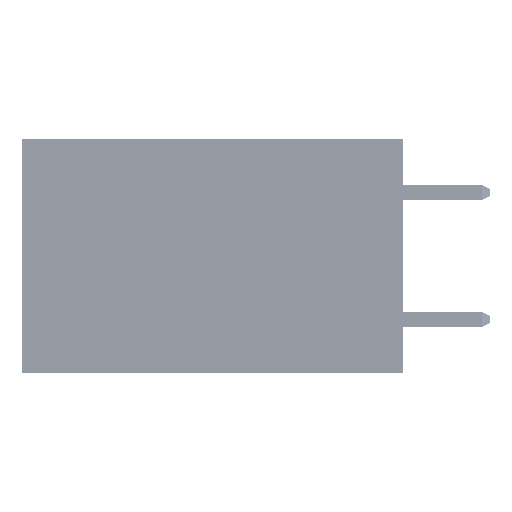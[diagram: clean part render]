
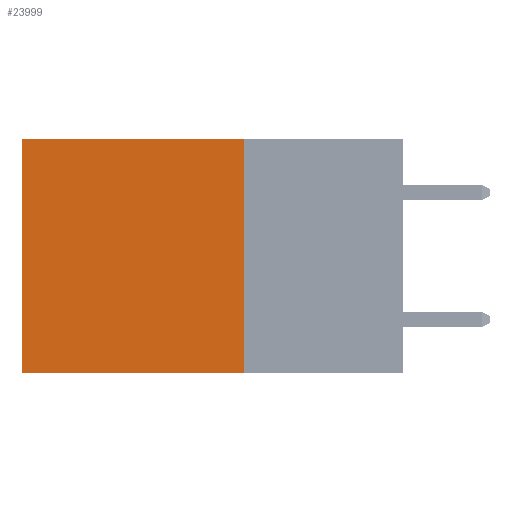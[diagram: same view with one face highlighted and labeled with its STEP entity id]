
A CAD part, left-side view. The second image highlights one B-rep face of the part: STEP entity #23999.
In plain terms, the highlighted planar face has unit normal (-1, 0, 0).
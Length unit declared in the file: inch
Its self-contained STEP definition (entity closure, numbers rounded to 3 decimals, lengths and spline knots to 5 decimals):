
#583 = EDGE_CURVE ( 'NONE', #38923, #5030, #13381, .T. ) ;
#1018 = DIRECTION ( 'NONE',  ( 0., 0., -1. ) ) ;
#1127 = DIRECTION ( 'NONE',  ( 0., 1., 0. ) ) ;
#1425 = CARTESIAN_POINT ( 'NONE',  ( 0.2875, 0.6, -0.37 ) ) ;
#4219 = ORIENTED_EDGE ( 'NONE', *, *, #45315, .T. ) ;
#4636 = ORIENTED_EDGE ( 'NONE', *, *, #12246, .T. ) ;
#5030 = VERTEX_POINT ( 'NONE', #37125 ) ;
#11521 = CARTESIAN_POINT ( 'NONE',  ( 0.2875, 0.6, 0. ) ) ;
#12246 = EDGE_CURVE ( 'NONE', #23086, #42691, #13013, .T. ) ;
#13013 = LINE ( 'NONE', #37591, #28903 ) ;
#13381 = LINE ( 'NONE', #17433, #22568 ) ;
#14791 = VECTOR ( 'NONE', #41757, 39.37008 ) ;
#17433 = CARTESIAN_POINT ( 'NONE',  ( 0.2875, 0.25, 0. ) ) ;
#17654 = DIRECTION ( 'NONE',  ( 0., 0., -1. ) ) ;
#18188 = ORIENTED_EDGE ( 'NONE', *, *, #583, .F. ) ;
#19488 = VECTOR ( 'NONE', #1127, 39.37008 ) ;
#19728 = FACE_OUTER_BOUND ( 'NONE', #33648, .T. ) ;
#22568 = VECTOR ( 'NONE', #35327, 39.37008 ) ;
#23086 = VERTEX_POINT ( 'NONE', #11521 ) ;
#23753 = LINE ( 'NONE', #39857, #19488 ) ;
#23999 = ADVANCED_FACE ( 'NONE', ( #19728 ), #36212, .F. ) ;
#24295 = EDGE_CURVE ( 'NONE', #5030, #42691, #39798, .T. ) ;
#24461 = DIRECTION ( 'NONE',  ( 1., 0., 0. ) ) ;
#28903 = VECTOR ( 'NONE', #17654, 39.37008 ) ;
#30183 = CARTESIAN_POINT ( 'NONE',  ( 0.2875, 0.25, 0. ) ) ;
#33388 = ORIENTED_EDGE ( 'NONE', *, *, #24295, .F. ) ;
#33648 = EDGE_LOOP ( 'NONE', ( #4636, #33388, #18188, #4219 ) ) ;
#35327 = DIRECTION ( 'NONE',  ( 0., 0., -1. ) ) ;
#36212 = PLANE ( 'NONE',  #38518 ) ;
#37125 = CARTESIAN_POINT ( 'NONE',  ( 0.2875, 0.25, -0.37 ) ) ;
#37591 = CARTESIAN_POINT ( 'NONE',  ( 0.2875, 0.6, 0. ) ) ;
#38518 = AXIS2_PLACEMENT_3D ( 'NONE', #47788, #24461, #1018 ) ;
#38923 = VERTEX_POINT ( 'NONE', #30183 ) ;
#39798 = LINE ( 'NONE', #42097, #14791 ) ;
#39857 = CARTESIAN_POINT ( 'NONE',  ( 0.2875, 0.25, 0. ) ) ;
#41757 = DIRECTION ( 'NONE',  ( 0., 1., 0. ) ) ;
#42097 = CARTESIAN_POINT ( 'NONE',  ( 0.2875, 0.25, -0.37 ) ) ;
#42691 = VERTEX_POINT ( 'NONE', #1425 ) ;
#45315 = EDGE_CURVE ( 'NONE', #38923, #23086, #23753, .T. ) ;
#47788 = CARTESIAN_POINT ( 'NONE',  ( 0.2875, 0.25, 0. ) ) ;
